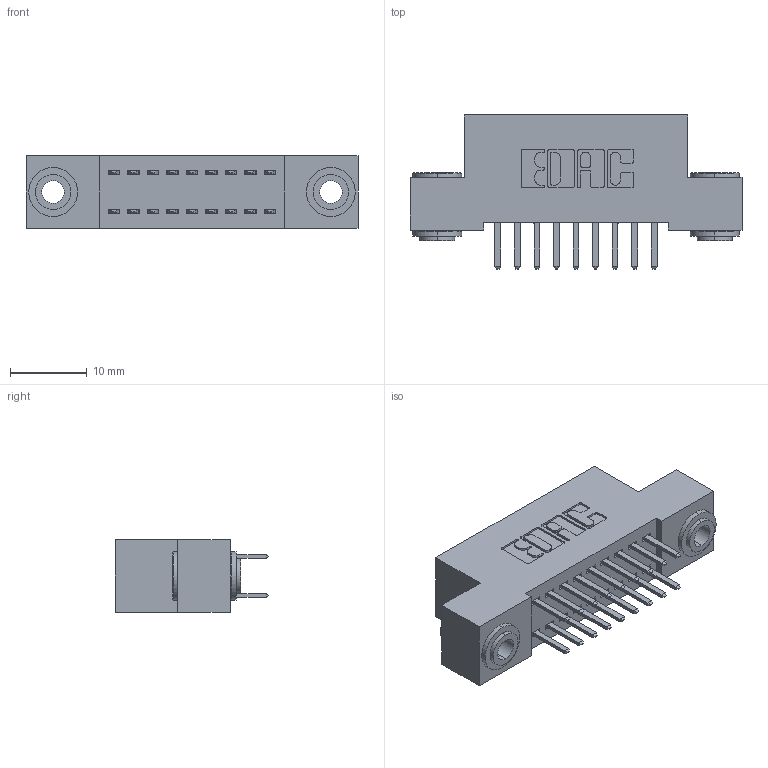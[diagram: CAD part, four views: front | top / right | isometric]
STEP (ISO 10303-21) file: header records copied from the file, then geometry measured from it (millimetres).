
FILE_DESCRIPTION (( 'STEP AP203' ), '1' );
FILE_NAME ('342-018-520-203.STEP', '2018-08-10T21:06:18', ( '' ), ( '' ), 'SwSTEP 2.0', 'SolidWorks 2016', '' );
FILE_SCHEMA (( 'CONFIG_CONTROL_DESIGN' ));
Length unit declared in the file: inch
Products named in the file (4): 345-292-001_345-293-120; 342-250-002_345-250-002-102; 342-018-520-203; 342 Part_.156 TH
Assembly tree (21 placements, depth 2):
  342-018-520-203
    342 Part_.156 TH
    345-292-001_345-293-120  x18
    342-250-002_345-250-002-102  x2
Bounding box: 43.18 x 20.02 x 9.4 mm (x, y, z)
Volume: 3738.4 mm3; surface area: 5467.5 mm2
Topology: 21 solids, 21 shells, 1156 faces, 3309 edges, 2154 vertices
Faces by surface type: plane 760, cylinder 388, cone 8
Entity records: 10690 total; most frequent: CARTESIAN_POINT 1797, ORIENTED_EDGE 1714, DIRECTION 1615, EDGE_CURVE 857, VECTOR 701, LINE 701, VERTEX_POINT 566, AXIS2_PLACEMENT_3D 457
